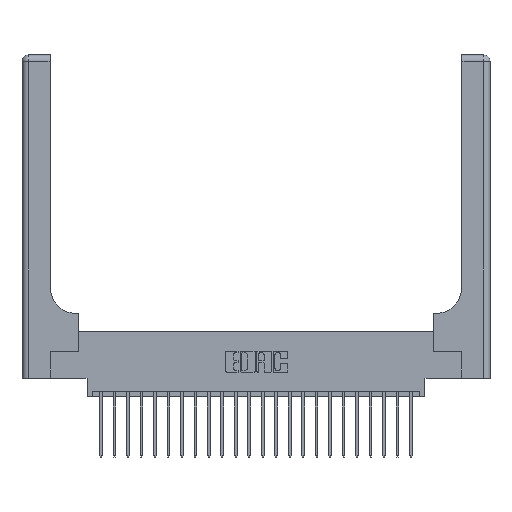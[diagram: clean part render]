
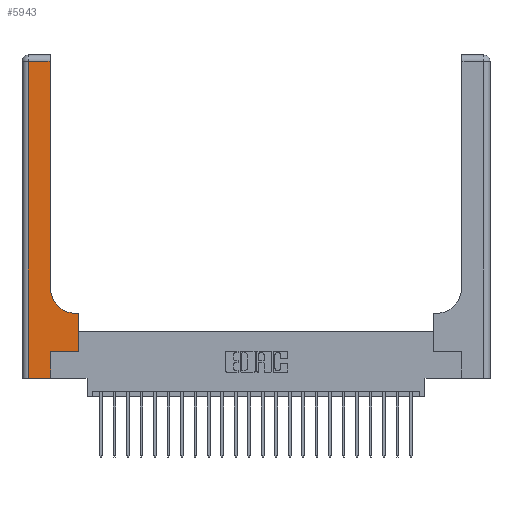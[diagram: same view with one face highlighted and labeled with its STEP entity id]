
A CAD part, top view. The second image highlights one B-rep face of the part: STEP entity #5943.
In plain terms, the highlighted planar face has unit normal (0, 0, 1).
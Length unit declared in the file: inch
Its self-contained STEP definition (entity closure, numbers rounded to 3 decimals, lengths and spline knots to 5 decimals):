
#203 = EDGE_CURVE ( 'NONE', #4452, #7406, #3233, .T. ) ;
#363 = CARTESIAN_POINT ( 'NONE',  ( 0.26, 3., 0.37 ) ) ;
#755 = DIRECTION ( 'NONE',  ( -1., 0., 0. ) ) ;
#943 = CARTESIAN_POINT ( 'NONE',  ( 0., 0., 0.37 ) ) ;
#1141 = CIRCLE ( 'NONE', #7908, 0.25 ) ;
#1993 = CARTESIAN_POINT ( 'NONE',  ( 0.06, 3., 0.37 ) ) ;
#2235 = EDGE_CURVE ( 'NONE', #3943, #18684, #12716, .T. ) ;
#2589 = EDGE_CURVE ( 'NONE', #7406, #6672, #1141, .T. ) ;
#2700 = VECTOR ( 'NONE', #11157, 39.37008 ) ;
#2963 = ORIENTED_EDGE ( 'NONE', *, *, #11799, .T. ) ;
#3233 = LINE ( 'NONE', #18247, #22513 ) ;
#3687 = LINE ( 'NONE', #22352, #22395 ) ;
#3784 = ORIENTED_EDGE ( 'NONE', *, *, #12254, .T. ) ;
#3943 = VERTEX_POINT ( 'NONE', #18433 ) ;
#4452 = VERTEX_POINT ( 'NONE', #17777 ) ;
#4589 = CARTESIAN_POINT ( 'NONE',  ( 0.265, 0., 0.37 ) ) ;
#4819 = DIRECTION ( 'NONE',  ( 0., 1., 0. ) ) ;
#5267 = EDGE_CURVE ( 'NONE', #18684, #4452, #3687, .T. ) ;
#5805 = AXIS2_PLACEMENT_3D ( 'NONE', #21570, #10677, #23375 ) ;
#5881 = VECTOR ( 'NONE', #21940, 39.37008 ) ;
#5943 = ADVANCED_FACE ( 'NONE', ( #17814 ), #19754, .F. ) ;
#6672 = VERTEX_POINT ( 'NONE', #13017 ) ;
#6795 = EDGE_CURVE ( 'NONE', #21488, #19501, #17770, .T. ) ;
#7406 = VERTEX_POINT ( 'NONE', #15685 ) ;
#7908 = AXIS2_PLACEMENT_3D ( 'NONE', #8824, #21511, #10617 ) ;
#7963 = VECTOR ( 'NONE', #17127, 39.37008 ) ;
#8390 = ORIENTED_EDGE ( 'NONE', *, *, #2589, .T. ) ;
#8824 = CARTESIAN_POINT ( 'NONE',  ( 0.51, 0.85, 0.37 ) ) ;
#8970 = ORIENTED_EDGE ( 'NONE', *, *, #2235, .T. ) ;
#9203 = DIRECTION ( 'NONE',  ( -1., 0., 0. ) ) ;
#9261 = VECTOR ( 'NONE', #13553, 39.37008 ) ;
#10617 = DIRECTION ( 'NONE',  ( 1., 0., 0. ) ) ;
#10660 = LINE ( 'NONE', #1993, #5881 ) ;
#10672 = EDGE_CURVE ( 'NONE', #19501, #3943, #19631, .T. ) ;
#10677 = DIRECTION ( 'NONE',  ( 0., 0., -1. ) ) ;
#11102 = ORIENTED_EDGE ( 'NONE', *, *, #10672, .T. ) ;
#11157 = DIRECTION ( 'NONE',  ( 0., 1., 0. ) ) ;
#11627 = VERTEX_POINT ( 'NONE', #20147 ) ;
#11712 = LINE ( 'NONE', #363, #2700 ) ;
#11799 = EDGE_CURVE ( 'NONE', #21259, #11627, #22695, .T. ) ;
#12254 = EDGE_CURVE ( 'NONE', #11627, #21488, #10660, .T. ) ;
#12400 = ORIENTED_EDGE ( 'NONE', *, *, #5267, .T. ) ;
#12423 = VECTOR ( 'NONE', #755, 39.37008 ) ;
#12716 = LINE ( 'NONE', #13433, #7963 ) ;
#12898 = ORIENTED_EDGE ( 'NONE', *, *, #203, .T. ) ;
#13017 = CARTESIAN_POINT ( 'NONE',  ( 0.26, 0.85, 0.37 ) ) ;
#13048 = CARTESIAN_POINT ( 'NONE',  ( 0.528, 0.25, 0.37 ) ) ;
#13433 = CARTESIAN_POINT ( 'NONE',  ( 0.265, 0.25, 0.37 ) ) ;
#13465 = EDGE_CURVE ( 'NONE', #6672, #21259, #11712, .T. ) ;
#13553 = DIRECTION ( 'NONE',  ( 1., 0., 0. ) ) ;
#15152 = ORIENTED_EDGE ( 'NONE', *, *, #6795, .T. ) ;
#15334 = ORIENTED_EDGE ( 'NONE', *, *, #13465, .T. ) ;
#15685 = CARTESIAN_POINT ( 'NONE',  ( 0.51, 0.6, 0.37 ) ) ;
#16969 = CARTESIAN_POINT ( 'NONE',  ( 0., 2.94, 0.37 ) ) ;
#17127 = DIRECTION ( 'NONE',  ( 1., 0., 0. ) ) ;
#17770 = LINE ( 'NONE', #943, #9261 ) ;
#17777 = CARTESIAN_POINT ( 'NONE',  ( 0.528, 0.6, 0.37 ) ) ;
#17814 = FACE_OUTER_BOUND ( 'NONE', #21422, .T. ) ;
#18247 = CARTESIAN_POINT ( 'NONE',  ( 0.26, 0.6, 0.37 ) ) ;
#18433 = CARTESIAN_POINT ( 'NONE',  ( 0.265, 0.25, 0.37 ) ) ;
#18684 = VERTEX_POINT ( 'NONE', #13048 ) ;
#18782 = DIRECTION ( 'NONE',  ( 0., 1., 0. ) ) ;
#18789 = CARTESIAN_POINT ( 'NONE',  ( 0.26, 2.94, 0.37 ) ) ;
#19056 = VECTOR ( 'NONE', #4819, 39.37008 ) ;
#19405 = CARTESIAN_POINT ( 'NONE',  ( 0.06, 0., 0.37 ) ) ;
#19501 = VERTEX_POINT ( 'NONE', #4589 ) ;
#19631 = LINE ( 'NONE', #22872, #19056 ) ;
#19754 = PLANE ( 'NONE',  #5805 ) ;
#20147 = CARTESIAN_POINT ( 'NONE',  ( 0.06, 2.94, 0.37 ) ) ;
#21259 = VERTEX_POINT ( 'NONE', #18789 ) ;
#21422 = EDGE_LOOP ( 'NONE', ( #15334, #2963, #3784, #15152, #11102, #8970, #12400, #12898, #8390 ) ) ;
#21488 = VERTEX_POINT ( 'NONE', #19405 ) ;
#21511 = DIRECTION ( 'NONE',  ( 0., 0., -1. ) ) ;
#21570 = CARTESIAN_POINT ( 'NONE',  ( 0., 3., 0.37 ) ) ;
#21940 = DIRECTION ( 'NONE',  ( 0., -1., 0. ) ) ;
#22352 = CARTESIAN_POINT ( 'NONE',  ( 0.528, 0.25, 0.37 ) ) ;
#22395 = VECTOR ( 'NONE', #18782, 39.37008 ) ;
#22513 = VECTOR ( 'NONE', #9203, 39.37008 ) ;
#22695 = LINE ( 'NONE', #16969, #12423 ) ;
#22872 = CARTESIAN_POINT ( 'NONE',  ( 0.265, 0., 0.37 ) ) ;
#23375 = DIRECTION ( 'NONE',  ( -1., 0., 0. ) ) ;
